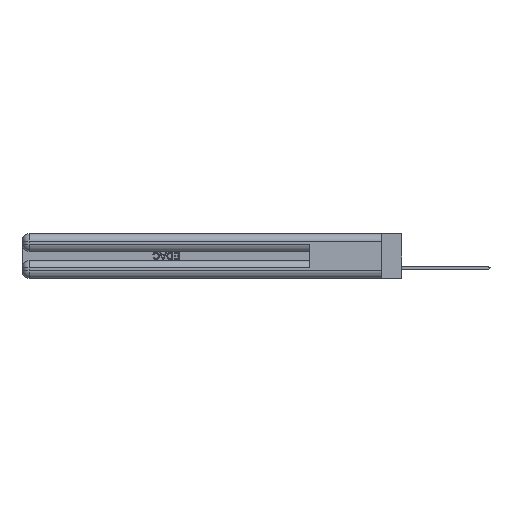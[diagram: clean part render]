
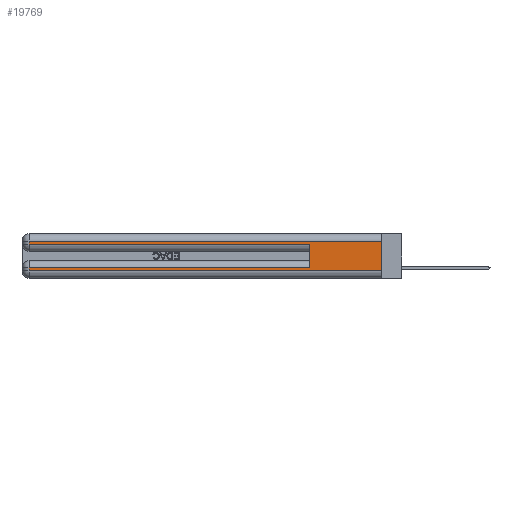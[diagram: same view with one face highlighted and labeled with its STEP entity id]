
A CAD part, left-side view. The second image highlights one B-rep face of the part: STEP entity #19769.
In plain terms, the highlighted planar face has unit normal (-1, 0, 0).
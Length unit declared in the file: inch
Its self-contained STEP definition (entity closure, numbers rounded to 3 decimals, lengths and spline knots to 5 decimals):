
#610 = VECTOR ( 'NONE', #17479, 39.37008 ) ;
#1425 = CARTESIAN_POINT ( 'NONE',  ( 0., 0., 0.085 ) ) ;
#1643 = VECTOR ( 'NONE', #29472, 39.37008 ) ;
#3184 = CARTESIAN_POINT ( 'NONE',  ( 0., 0.6, 0.285 ) ) ;
#3563 = VERTEX_POINT ( 'NONE', #20484 ) ;
#3778 = CARTESIAN_POINT ( 'NONE',  ( 0., 2.94, 0.31 ) ) ;
#3866 = VECTOR ( 'NONE', #5840, 39.37008 ) ;
#4546 = DIRECTION ( 'NONE',  ( 0., 1., 0. ) ) ;
#4904 = VECTOR ( 'NONE', #28393, 39.37008 ) ;
#5840 = DIRECTION ( 'NONE',  ( 0., -1., 0. ) ) ;
#6994 = EDGE_CURVE ( 'NONE', #14047, #14549, #32617, .T. ) ;
#9512 = EDGE_CURVE ( 'NONE', #14549, #32845, #16964, .T. ) ;
#9605 = EDGE_LOOP ( 'NONE', ( #10271, #30699, #23581, #32871, #20782, #29587, #38878, #16189 ) ) ;
#10271 = ORIENTED_EDGE ( 'NONE', *, *, #29923, .F. ) ;
#10563 = LINE ( 'NONE', #37378, #4904 ) ;
#11232 = PLANE ( 'NONE',  #23558 ) ;
#11484 = VECTOR ( 'NONE', #38896, 39.37008 ) ;
#11542 = CARTESIAN_POINT ( 'NONE',  ( 0., 2.94, 0.37 ) ) ;
#13656 = FACE_OUTER_BOUND ( 'NONE', #9605, .T. ) ;
#13997 = VECTOR ( 'NONE', #4546, 39.37008 ) ;
#14047 = VERTEX_POINT ( 'NONE', #28252 ) ;
#14109 = VECTOR ( 'NONE', #34028, 39.37008 ) ;
#14549 = VERTEX_POINT ( 'NONE', #3778 ) ;
#15761 = DIRECTION ( 'NONE',  ( 0., 1., 0. ) ) ;
#16167 = VECTOR ( 'NONE', #15761, 39.37008 ) ;
#16189 = ORIENTED_EDGE ( 'NONE', *, *, #35092, .T. ) ;
#16964 = LINE ( 'NONE', #29606, #1643 ) ;
#17410 = DIRECTION ( 'NONE',  ( 1., 0., 0. ) ) ;
#17479 = DIRECTION ( 'NONE',  ( 0., 0., -1. ) ) ;
#19662 = LINE ( 'NONE', #11542, #11484 ) ;
#19769 = ADVANCED_FACE ( 'NONE', ( #13656 ), #11232, .F. ) ;
#20049 = CARTESIAN_POINT ( 'NONE',  ( 0., 2.94, 0.285 ) ) ;
#20206 = CARTESIAN_POINT ( 'NONE',  ( 0., 2.94, 0.085 ) ) ;
#20484 = CARTESIAN_POINT ( 'NONE',  ( 0., 0., 0.06 ) ) ;
#20699 = VERTEX_POINT ( 'NONE', #22681 ) ;
#20782 = ORIENTED_EDGE ( 'NONE', *, *, #35211, .F. ) ;
#22681 = CARTESIAN_POINT ( 'NONE',  ( 0., 2.94, 0.06 ) ) ;
#23558 = AXIS2_PLACEMENT_3D ( 'NONE', #35896, #17410, #29981 ) ;
#23581 = ORIENTED_EDGE ( 'NONE', *, *, #9512, .T. ) ;
#24556 = VERTEX_POINT ( 'NONE', #20206 ) ;
#25024 = CARTESIAN_POINT ( 'NONE',  ( 0., 0.6, 0.145 ) ) ;
#26194 = CARTESIAN_POINT ( 'NONE',  ( 0., 0.6, 0.085 ) ) ;
#27905 = EDGE_CURVE ( 'NONE', #32845, #30992, #10563, .T. ) ;
#28252 = CARTESIAN_POINT ( 'NONE',  ( 0., 0., 0.31 ) ) ;
#28393 = DIRECTION ( 'NONE',  ( 0., -1., 0. ) ) ;
#29472 = DIRECTION ( 'NONE',  ( 0., 0., -1. ) ) ;
#29587 = ORIENTED_EDGE ( 'NONE', *, *, #30789, .T. ) ;
#29606 = CARTESIAN_POINT ( 'NONE',  ( 0., 2.94, 0.37 ) ) ;
#29923 = EDGE_CURVE ( 'NONE', #14047, #3563, #33391, .T. ) ;
#29981 = DIRECTION ( 'NONE',  ( 0., 0., -1. ) ) ;
#30699 = ORIENTED_EDGE ( 'NONE', *, *, #6994, .T. ) ;
#30789 = EDGE_CURVE ( 'NONE', #36761, #24556, #35720, .T. ) ;
#30992 = VERTEX_POINT ( 'NONE', #3184 ) ;
#32617 = LINE ( 'NONE', #34114, #16167 ) ;
#32837 = CARTESIAN_POINT ( 'NONE',  ( 0., 0., 0.37 ) ) ;
#32845 = VERTEX_POINT ( 'NONE', #20049 ) ;
#32871 = ORIENTED_EDGE ( 'NONE', *, *, #27905, .T. ) ;
#32943 = EDGE_CURVE ( 'NONE', #24556, #20699, #19662, .T. ) ;
#33391 = LINE ( 'NONE', #32837, #610 ) ;
#34028 = DIRECTION ( 'NONE',  ( 0., 0., 1. ) ) ;
#34114 = CARTESIAN_POINT ( 'NONE',  ( 0., 0., 0.31 ) ) ;
#35092 = EDGE_CURVE ( 'NONE', #20699, #3563, #35123, .T. ) ;
#35123 = LINE ( 'NONE', #36510, #3866 ) ;
#35211 = EDGE_CURVE ( 'NONE', #36761, #30992, #39745, .T. ) ;
#35720 = LINE ( 'NONE', #1425, #13997 ) ;
#35896 = CARTESIAN_POINT ( 'NONE',  ( 0., 0., 0.37 ) ) ;
#36510 = CARTESIAN_POINT ( 'NONE',  ( 0., 0., 0.06 ) ) ;
#36761 = VERTEX_POINT ( 'NONE', #26194 ) ;
#37378 = CARTESIAN_POINT ( 'NONE',  ( 0., 0., 0.285 ) ) ;
#38878 = ORIENTED_EDGE ( 'NONE', *, *, #32943, .T. ) ;
#38896 = DIRECTION ( 'NONE',  ( 0., 0., -1. ) ) ;
#39745 = LINE ( 'NONE', #25024, #14109 ) ;
